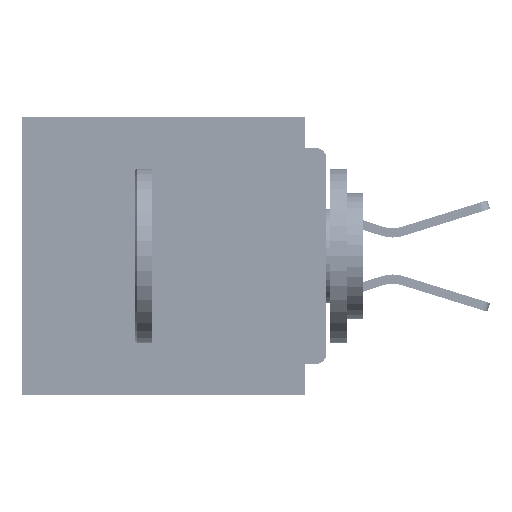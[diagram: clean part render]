
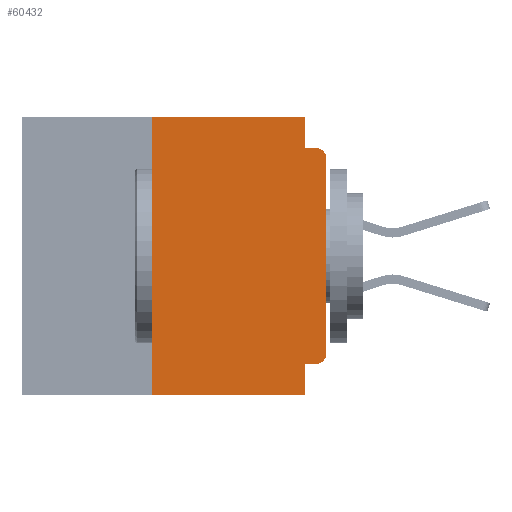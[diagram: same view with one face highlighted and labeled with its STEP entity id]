
A CAD part, left-side view. The second image highlights one B-rep face of the part: STEP entity #60432.
In plain terms, the highlighted planar face has unit normal (-1, 0, 0).
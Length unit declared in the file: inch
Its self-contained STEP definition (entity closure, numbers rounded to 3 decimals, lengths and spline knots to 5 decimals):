
#56 = VERTEX_POINT ( 'NONE', #66252 ) ;
#120 = CIRCLE ( 'NONE', #50726, 0.015 ) ;
#282 = ORIENTED_EDGE ( 'NONE', *, *, #20555, .T. ) ;
#624 = VECTOR ( 'NONE', #16978, 39.37008 ) ;
#1137 = DIRECTION ( 'NONE',  ( -1., 0., 0. ) ) ;
#1333 = ORIENTED_EDGE ( 'NONE', *, *, #24820, .F. ) ;
#2035 = CARTESIAN_POINT ( 'NONE',  ( 0., 0.031, -0.045 ) ) ;
#2523 = AXIS2_PLACEMENT_3D ( 'NONE', #34255, #1137, #39820 ) ;
#2553 = AXIS2_PLACEMENT_3D ( 'NONE', #15728, #54263, #21308 ) ;
#4803 = EDGE_CURVE ( 'NONE', #67032, #66731, #59412, .T. ) ;
#7361 = VECTOR ( 'NONE', #55466, 39.37008 ) ;
#7933 = LINE ( 'NONE', #18329, #64849 ) ;
#8178 = FACE_OUTER_BOUND ( 'NONE', #45886, .T. ) ;
#8363 = CARTESIAN_POINT ( 'NONE',  ( 0., 0.031, -0.4 ) ) ;
#8963 = EDGE_CURVE ( 'NONE', #53222, #53899, #50158, .T. ) ;
#9735 = VECTOR ( 'NONE', #13943, 39.37008 ) ;
#10568 = ORIENTED_EDGE ( 'NONE', *, *, #48091, .F. ) ;
#11364 = CARTESIAN_POINT ( 'NONE',  ( 0., 0.015, -0.06 ) ) ;
#12230 = ORIENTED_EDGE ( 'NONE', *, *, #65193, .F. ) ;
#12905 = CARTESIAN_POINT ( 'NONE',  ( 0., 0.25, -0.4 ) ) ;
#13457 = ORIENTED_EDGE ( 'NONE', *, *, #8963, .T. ) ;
#13545 = CARTESIAN_POINT ( 'NONE',  ( 0., 0.031, -0.4 ) ) ;
#13943 = DIRECTION ( 'NONE',  ( 0., 0., -1. ) ) ;
#14124 = CARTESIAN_POINT ( 'NONE',  ( 0., 0., 0. ) ) ;
#14720 = CIRCLE ( 'NONE', #2523, 0.015 ) ;
#14828 = CARTESIAN_POINT ( 'NONE',  ( 0., 0.437, -0.4 ) ) ;
#15728 = CARTESIAN_POINT ( 'NONE',  ( 0., 0.437, 0. ) ) ;
#16881 = DIRECTION ( 'NONE',  ( 0., 0., -1. ) ) ;
#16978 = DIRECTION ( 'NONE',  ( 0., 1., 0. ) ) ;
#18329 = CARTESIAN_POINT ( 'NONE',  ( 0., 0.437, 0. ) ) ;
#19548 = VERTEX_POINT ( 'NONE', #24552 ) ;
#19687 = LINE ( 'NONE', #55150, #50659 ) ;
#20555 = EDGE_CURVE ( 'NONE', #19548, #67032, #14720, .T. ) ;
#21308 = DIRECTION ( 'NONE',  ( 0., 0., -1. ) ) ;
#22199 = DIRECTION ( 'NONE',  ( 0., -1., 0. ) ) ;
#22806 = CARTESIAN_POINT ( 'NONE',  ( 0., 0., -0.355 ) ) ;
#23867 = LINE ( 'NONE', #28066, #7361 ) ;
#24552 = CARTESIAN_POINT ( 'NONE',  ( 0., 0.015, -0.355 ) ) ;
#24820 = EDGE_CURVE ( 'NONE', #61392, #34507, #19687, .T. ) ;
#25220 = CARTESIAN_POINT ( 'NONE',  ( 0., 0.015, -0.045 ) ) ;
#28066 = CARTESIAN_POINT ( 'NONE',  ( 0., 0.031, 0. ) ) ;
#31757 = CARTESIAN_POINT ( 'NONE',  ( 0., 0., -0.06 ) ) ;
#32107 = VECTOR ( 'NONE', #42355, 39.37008 ) ;
#34164 = CARTESIAN_POINT ( 'NONE',  ( 0., 0.25, -0.4 ) ) ;
#34255 = CARTESIAN_POINT ( 'NONE',  ( 0., 0.015, -0.34 ) ) ;
#34507 = VERTEX_POINT ( 'NONE', #25220 ) ;
#34729 = DIRECTION ( 'NONE',  ( 0., -1., 0. ) ) ;
#35498 = EDGE_CURVE ( 'NONE', #53222, #57431, #54599, .T. ) ;
#36036 = VERTEX_POINT ( 'NONE', #71310 ) ;
#38277 = VECTOR ( 'NONE', #56037, 39.37008 ) ;
#39820 = DIRECTION ( 'NONE',  ( 0., 0., -1. ) ) ;
#42355 = DIRECTION ( 'NONE',  ( 0., -1., 0. ) ) ;
#43395 = EDGE_CURVE ( 'NONE', #57431, #56, #7933, .T. ) ;
#44223 = ORIENTED_EDGE ( 'NONE', *, *, #43395, .F. ) ;
#44694 = CARTESIAN_POINT ( 'NONE',  ( 0., 0.25, 0. ) ) ;
#45700 = CARTESIAN_POINT ( 'NONE',  ( 0., 0., -0.34 ) ) ;
#45886 = EDGE_LOOP ( 'NONE', ( #55954, #45925, #1333, #53992, #44223, #50122, #13457, #10568, #12230, #282 ) ) ;
#45925 = ORIENTED_EDGE ( 'NONE', *, *, #62824, .T. ) ;
#46893 = EDGE_CURVE ( 'NONE', #56, #61392, #23867, .T. ) ;
#48091 = EDGE_CURVE ( 'NONE', #36036, #53899, #53706, .T. ) ;
#48746 = PLANE ( 'NONE',  #2553 ) ;
#49899 = DIRECTION ( 'NONE',  ( -1., 0., 0. ) ) ;
#50122 = ORIENTED_EDGE ( 'NONE', *, *, #35498, .F. ) ;
#50158 = LINE ( 'NONE', #14828, #32107 ) ;
#50659 = VECTOR ( 'NONE', #22199, 39.37008 ) ;
#50726 = AXIS2_PLACEMENT_3D ( 'NONE', #11364, #49899, #16881 ) ;
#53222 = VERTEX_POINT ( 'NONE', #12905 ) ;
#53706 = LINE ( 'NONE', #8363, #9735 ) ;
#53899 = VERTEX_POINT ( 'NONE', #13545 ) ;
#53992 = ORIENTED_EDGE ( 'NONE', *, *, #46893, .F. ) ;
#54263 = DIRECTION ( 'NONE',  ( 1., 0., 0. ) ) ;
#54599 = LINE ( 'NONE', #34164, #38277 ) ;
#55150 = CARTESIAN_POINT ( 'NONE',  ( 0., 0., -0.045 ) ) ;
#55466 = DIRECTION ( 'NONE',  ( 0., 0., -1. ) ) ;
#55954 = ORIENTED_EDGE ( 'NONE', *, *, #4803, .T. ) ;
#56037 = DIRECTION ( 'NONE',  ( 0., 0., 1. ) ) ;
#57431 = VERTEX_POINT ( 'NONE', #44694 ) ;
#57567 = LINE ( 'NONE', #22806, #624 ) ;
#57682 = VECTOR ( 'NONE', #63726, 39.37008 ) ;
#59412 = LINE ( 'NONE', #14124, #57682 ) ;
#60432 = ADVANCED_FACE ( 'NONE', ( #8178 ), #48746, .F. ) ;
#61392 = VERTEX_POINT ( 'NONE', #2035 ) ;
#62824 = EDGE_CURVE ( 'NONE', #66731, #34507, #120, .T. ) ;
#63726 = DIRECTION ( 'NONE',  ( 0., 0., 1. ) ) ;
#64849 = VECTOR ( 'NONE', #34729, 39.37008 ) ;
#65193 = EDGE_CURVE ( 'NONE', #19548, #36036, #57567, .T. ) ;
#66252 = CARTESIAN_POINT ( 'NONE',  ( 0., 0.031, 0. ) ) ;
#66731 = VERTEX_POINT ( 'NONE', #31757 ) ;
#67032 = VERTEX_POINT ( 'NONE', #45700 ) ;
#71310 = CARTESIAN_POINT ( 'NONE',  ( 0., 0.031, -0.355 ) ) ;
